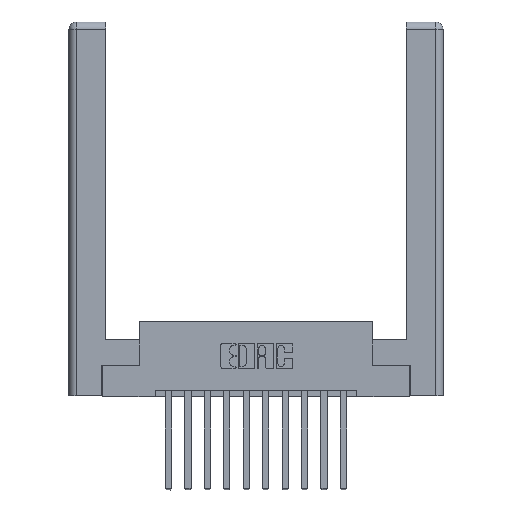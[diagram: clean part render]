
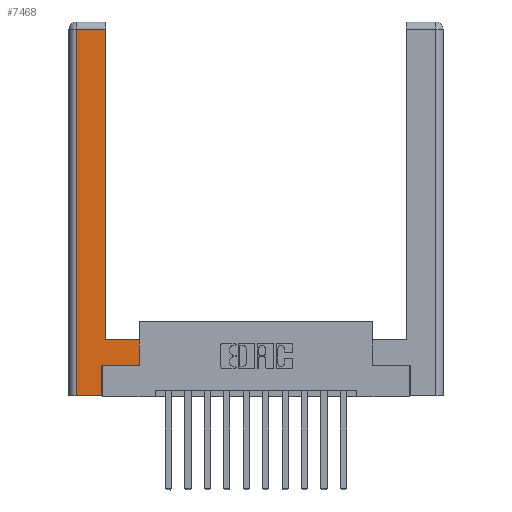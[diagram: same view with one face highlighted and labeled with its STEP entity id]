
A CAD part, top view. The second image highlights one B-rep face of the part: STEP entity #7468.
In plain terms, the highlighted planar face has unit normal (0, 0, 1).
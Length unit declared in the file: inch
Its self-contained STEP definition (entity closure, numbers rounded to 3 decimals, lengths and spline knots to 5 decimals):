
#184 = VERTEX_POINT ( 'NONE', #1588 ) ;
#222 = DIRECTION ( 'NONE',  ( 0., 1., 0. ) ) ;
#252 = ORIENTED_EDGE ( 'NONE', *, *, #9932, .T. ) ;
#447 = DIRECTION ( 'NONE',  ( 0., 1., 0. ) ) ;
#500 = VERTEX_POINT ( 'NONE', #8667 ) ;
#584 = CARTESIAN_POINT ( 'NONE',  ( 0.265, 0., 0. ) ) ;
#916 = VERTEX_POINT ( 'NONE', #5113 ) ;
#1298 = DIRECTION ( 'NONE',  ( -1., 0., 0. ) ) ;
#1335 = VERTEX_POINT ( 'NONE', #11357 ) ;
#1588 = CARTESIAN_POINT ( 'NONE',  ( 0.0615, 2.94, 0. ) ) ;
#1924 = LINE ( 'NONE', #3634, #3837 ) ;
#2023 = EDGE_CURVE ( 'NONE', #12589, #5888, #2169, .T. ) ;
#2133 = CARTESIAN_POINT ( 'NONE',  ( 0.295, 3., 0. ) ) ;
#2169 = LINE ( 'NONE', #7286, #3220 ) ;
#2237 = EDGE_CURVE ( 'NONE', #1335, #916, #12063, .T. ) ;
#2480 = CARTESIAN_POINT ( 'NONE',  ( 0.0615, 0., 0. ) ) ;
#3136 = EDGE_CURVE ( 'NONE', #12181, #12589, #10828, .T. ) ;
#3187 = EDGE_CURVE ( 'NONE', #5888, #3674, #3711, .T. ) ;
#3220 = VECTOR ( 'NONE', #12859, 39.37008 ) ;
#3253 = DIRECTION ( 'NONE',  ( -1., 0., 0. ) ) ;
#3631 = ORIENTED_EDGE ( 'NONE', *, *, #11322, .T. ) ;
#3634 = CARTESIAN_POINT ( 'NONE',  ( 0.295, 0.45, 0. ) ) ;
#3674 = VERTEX_POINT ( 'NONE', #13474 ) ;
#3711 = LINE ( 'NONE', #11415, #13240 ) ;
#3837 = VECTOR ( 'NONE', #1298, 39.37008 ) ;
#3959 = ORIENTED_EDGE ( 'NONE', *, *, #10052, .T. ) ;
#4288 = CARTESIAN_POINT ( 'NONE',  ( 0.265, 0.245, 0. ) ) ;
#4306 = ORIENTED_EDGE ( 'NONE', *, *, #2237, .T. ) ;
#4579 = ORIENTED_EDGE ( 'NONE', *, *, #3187, .T. ) ;
#4808 = DIRECTION ( 'NONE',  ( 0., -1., 0. ) ) ;
#5113 = CARTESIAN_POINT ( 'NONE',  ( 0.295, 2.94, 0. ) ) ;
#5316 = EDGE_CURVE ( 'NONE', #916, #184, #6764, .T. ) ;
#5346 = DIRECTION ( 'NONE',  ( 0., 0., -1. ) ) ;
#5540 = VECTOR ( 'NONE', #4808, 39.37008 ) ;
#5888 = VERTEX_POINT ( 'NONE', #12937 ) ;
#5948 = VECTOR ( 'NONE', #7568, 39.37008 ) ;
#6174 = AXIS2_PLACEMENT_3D ( 'NONE', #8637, #5346, #3253 ) ;
#6187 = DIRECTION ( 'NONE',  ( -1., 0., 0. ) ) ;
#6438 = EDGE_LOOP ( 'NONE', ( #4306, #14079, #3631, #252, #6751, #9189, #4579, #3959 ) ) ;
#6678 = VECTOR ( 'NONE', #9702, 39.37008 ) ;
#6751 = ORIENTED_EDGE ( 'NONE', *, *, #3136, .T. ) ;
#6764 = LINE ( 'NONE', #12806, #9032 ) ;
#7174 = VECTOR ( 'NONE', #222, 39.37008 ) ;
#7286 = CARTESIAN_POINT ( 'NONE',  ( 0.565, 0.245, 0. ) ) ;
#7468 = ADVANCED_FACE ( 'NONE', ( #8977 ), #8839, .F. ) ;
#7568 = DIRECTION ( 'NONE',  ( 1., 0., 0. ) ) ;
#8637 = CARTESIAN_POINT ( 'NONE',  ( 0., 0., 0. ) ) ;
#8667 = CARTESIAN_POINT ( 'NONE',  ( 0.0615, 0., 0. ) ) ;
#8839 = PLANE ( 'NONE',  #6174 ) ;
#8977 = FACE_OUTER_BOUND ( 'NONE', #6438, .T. ) ;
#9032 = VECTOR ( 'NONE', #6187, 39.37008 ) ;
#9189 = ORIENTED_EDGE ( 'NONE', *, *, #2023, .T. ) ;
#9702 = DIRECTION ( 'NONE',  ( 0., 1., 0. ) ) ;
#9932 = EDGE_CURVE ( 'NONE', #500, #12181, #12699, .T. ) ;
#10052 = EDGE_CURVE ( 'NONE', #3674, #1335, #1924, .T. ) ;
#10828 = LINE ( 'NONE', #4288, #7174 ) ;
#11322 = EDGE_CURVE ( 'NONE', #184, #500, #11929, .T. ) ;
#11357 = CARTESIAN_POINT ( 'NONE',  ( 0.295, 0.45, 0. ) ) ;
#11415 = CARTESIAN_POINT ( 'NONE',  ( 0.565, 0.45, 0. ) ) ;
#11929 = LINE ( 'NONE', #2480, #5540 ) ;
#12063 = LINE ( 'NONE', #2133, #6678 ) ;
#12181 = VERTEX_POINT ( 'NONE', #13012 ) ;
#12521 = CARTESIAN_POINT ( 'NONE',  ( 0.265, 0.245, 0. ) ) ;
#12589 = VERTEX_POINT ( 'NONE', #12521 ) ;
#12699 = LINE ( 'NONE', #584, #5948 ) ;
#12806 = CARTESIAN_POINT ( 'NONE',  ( 0.0615, 2.94, 0. ) ) ;
#12859 = DIRECTION ( 'NONE',  ( 1., 0., 0. ) ) ;
#12937 = CARTESIAN_POINT ( 'NONE',  ( 0.565, 0.245, 0. ) ) ;
#13012 = CARTESIAN_POINT ( 'NONE',  ( 0.265, 0., 0. ) ) ;
#13240 = VECTOR ( 'NONE', #447, 39.37008 ) ;
#13474 = CARTESIAN_POINT ( 'NONE',  ( 0.565, 0.45, 0. ) ) ;
#14079 = ORIENTED_EDGE ( 'NONE', *, *, #5316, .T. ) ;
